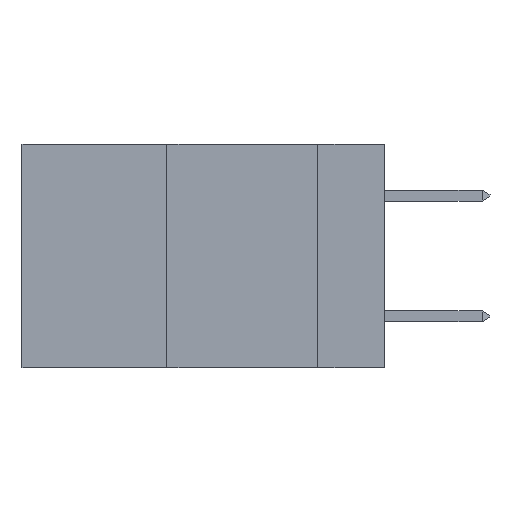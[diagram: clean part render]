
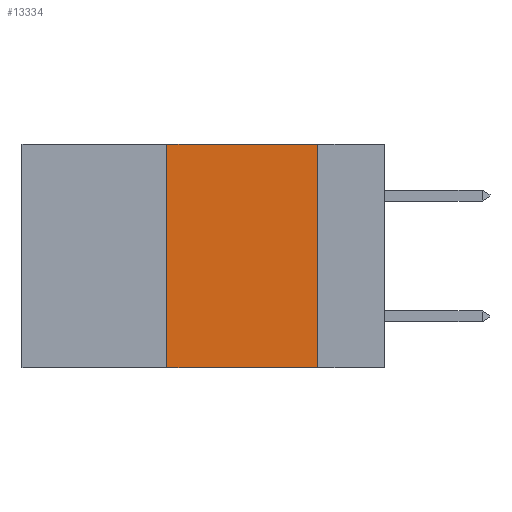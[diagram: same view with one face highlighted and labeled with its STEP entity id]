
A CAD part, left-side view. The second image highlights one B-rep face of the part: STEP entity #13334.
In plain terms, the highlighted planar face has unit normal (-1, 0, 0).
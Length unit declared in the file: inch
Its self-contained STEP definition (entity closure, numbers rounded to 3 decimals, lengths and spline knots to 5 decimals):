
#3 = CARTESIAN_POINT ( 'NONE',  ( 0., 0.11, -0.37 ) ) ;
#1192 = CARTESIAN_POINT ( 'NONE',  ( 0., 0.6, 0. ) ) ;
#1317 = VECTOR ( 'NONE', #12473, 39.37008 ) ;
#1647 = CARTESIAN_POINT ( 'NONE',  ( 0., 0.6, 0. ) ) ;
#1910 = EDGE_LOOP ( 'NONE', ( #6562, #6642, #6723, #6988 ) ) ;
#2736 = DIRECTION ( 'NONE',  ( 0., 0., -1. ) ) ;
#2774 = VERTEX_POINT ( 'NONE', #2999 ) ;
#2999 = CARTESIAN_POINT ( 'NONE',  ( 0., 0.36, -0.37 ) ) ;
#3110 = DIRECTION ( 'NONE',  ( 0., 0., 1. ) ) ;
#3386 = EDGE_CURVE ( 'NONE', #2774, #5659, #4552, .T. ) ;
#3687 = VECTOR ( 'NONE', #12646, 39.37008 ) ;
#4404 = CARTESIAN_POINT ( 'NONE',  ( 0., 0.11, 0. ) ) ;
#4552 = LINE ( 'NONE', #9198, #1317 ) ;
#4860 = PLANE ( 'NONE',  #7272 ) ;
#5038 = EDGE_CURVE ( 'NONE', #9307, #10602, #11836, .T. ) ;
#5659 = VERTEX_POINT ( 'NONE', #3 ) ;
#6234 = CARTESIAN_POINT ( 'NONE',  ( 0., 0.36, 0. ) ) ;
#6562 = ORIENTED_EDGE ( 'NONE', *, *, #11592, .F. ) ;
#6642 = ORIENTED_EDGE ( 'NONE', *, *, #5038, .F. ) ;
#6723 = ORIENTED_EDGE ( 'NONE', *, *, #8046, .F. ) ;
#6988 = ORIENTED_EDGE ( 'NONE', *, *, #3386, .T. ) ;
#7014 = DIRECTION ( 'NONE',  ( 0., 0., -1. ) ) ;
#7272 = AXIS2_PLACEMENT_3D ( 'NONE', #1647, #8921, #2736 ) ;
#8022 = CARTESIAN_POINT ( 'NONE',  ( 0., 0.11, 0. ) ) ;
#8046 = EDGE_CURVE ( 'NONE', #2774, #9307, #13395, .T. ) ;
#8436 = VECTOR ( 'NONE', #7014, 39.37008 ) ;
#8921 = DIRECTION ( 'NONE',  ( 1., 0., 0. ) ) ;
#9198 = CARTESIAN_POINT ( 'NONE',  ( 0., 0.6, -0.37 ) ) ;
#9307 = VERTEX_POINT ( 'NONE', #10432 ) ;
#9373 = FACE_OUTER_BOUND ( 'NONE', #1910, .T. ) ;
#10432 = CARTESIAN_POINT ( 'NONE',  ( 0., 0.36, 0. ) ) ;
#10602 = VERTEX_POINT ( 'NONE', #4404 ) ;
#10976 = VECTOR ( 'NONE', #3110, 39.37008 ) ;
#11197 = LINE ( 'NONE', #8022, #8436 ) ;
#11592 = EDGE_CURVE ( 'NONE', #10602, #5659, #11197, .T. ) ;
#11836 = LINE ( 'NONE', #1192, #3687 ) ;
#12473 = DIRECTION ( 'NONE',  ( 0., -1., 0. ) ) ;
#12646 = DIRECTION ( 'NONE',  ( 0., -1., 0. ) ) ;
#13334 = ADVANCED_FACE ( 'NONE', ( #9373 ), #4860, .F. ) ;
#13395 = LINE ( 'NONE', #6234, #10976 ) ;
